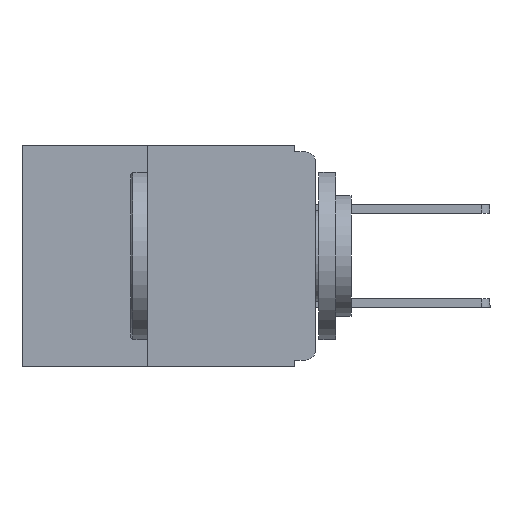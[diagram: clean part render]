
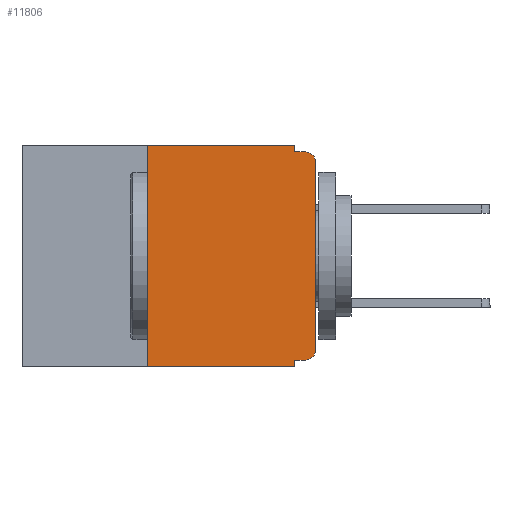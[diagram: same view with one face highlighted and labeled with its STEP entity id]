
A CAD part, left-side view. The second image highlights one B-rep face of the part: STEP entity #11806.
In plain terms, the highlighted planar face has unit normal (-1, 0, 0).
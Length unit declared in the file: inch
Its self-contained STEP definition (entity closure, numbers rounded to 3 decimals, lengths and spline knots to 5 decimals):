
#824 = EDGE_CURVE ( 'NONE', #16951, #5753, #6461, .T. ) ;
#980 = DIRECTION ( 'NONE',  ( 0., -1., 0. ) ) ;
#1070 = CARTESIAN_POINT ( 'NONE',  ( 0., 0., -0.305 ) ) ;
#1352 = EDGE_CURVE ( 'NONE', #15183, #16943, #2211, .T. ) ;
#1649 = VERTEX_POINT ( 'NONE', #15265 ) ;
#1796 = EDGE_CURVE ( 'NONE', #6173, #6223, #10322, .T. ) ;
#1927 = ORIENTED_EDGE ( 'NONE', *, *, #824, .F. ) ;
#2012 = VERTEX_POINT ( 'NONE', #11106 ) ;
#2022 = DIRECTION ( 'NONE',  ( 0., 0., -1. ) ) ;
#2211 = CIRCLE ( 'NONE', #7784, 0.015 ) ;
#2350 = VECTOR ( 'NONE', #8326, 39.37008 ) ;
#2513 = LINE ( 'NONE', #5973, #13495 ) ;
#2832 = VECTOR ( 'NONE', #980, 39.37008 ) ;
#3744 = EDGE_CURVE ( 'NONE', #2012, #5484, #15896, .T. ) ;
#3760 = ORIENTED_EDGE ( 'NONE', *, *, #16288, .F. ) ;
#3963 = ORIENTED_EDGE ( 'NONE', *, *, #9314, .F. ) ;
#4223 = CARTESIAN_POINT ( 'NONE',  ( 0., 0.437, -0.33 ) ) ;
#4314 = AXIS2_PLACEMENT_3D ( 'NONE', #6509, #6327, #6325 ) ;
#4913 = CARTESIAN_POINT ( 'NONE',  ( 0., 0.031, -0.32 ) ) ;
#5142 = ORIENTED_EDGE ( 'NONE', *, *, #7722, .F. ) ;
#5484 = VERTEX_POINT ( 'NONE', #10378 ) ;
#5493 = CARTESIAN_POINT ( 'NONE',  ( 0., 0., -0.32 ) ) ;
#5753 = VERTEX_POINT ( 'NONE', #10922 ) ;
#5779 = DIRECTION ( 'NONE',  ( 0., 0., 1. ) ) ;
#5806 = EDGE_CURVE ( 'NONE', #16943, #6173, #2513, .T. ) ;
#5818 = CARTESIAN_POINT ( 'NONE',  ( 0., 0.031, -0.33 ) ) ;
#5973 = CARTESIAN_POINT ( 'NONE',  ( 0., 0., 0. ) ) ;
#6000 = VECTOR ( 'NONE', #6075, 39.37008 ) ;
#6075 = DIRECTION ( 'NONE',  ( 0., 0., -1. ) ) ;
#6167 = VECTOR ( 'NONE', #16629, 39.37008 ) ;
#6173 = VERTEX_POINT ( 'NONE', #9390 ) ;
#6223 = VERTEX_POINT ( 'NONE', #9029 ) ;
#6226 = ORIENTED_EDGE ( 'NONE', *, *, #9392, .T. ) ;
#6325 = DIRECTION ( 'NONE',  ( 0., 0., -1. ) ) ;
#6327 = DIRECTION ( 'NONE',  ( -1., 0., 0. ) ) ;
#6461 = LINE ( 'NONE', #13357, #13639 ) ;
#6509 = CARTESIAN_POINT ( 'NONE',  ( 0., 0.015, -0.025 ) ) ;
#7722 = EDGE_CURVE ( 'NONE', #15510, #1649, #13208, .T. ) ;
#7759 = DIRECTION ( 'NONE',  ( -1., 0., 0. ) ) ;
#7763 = DIRECTION ( 'NONE',  ( 0., -1., 0. ) ) ;
#7784 = AXIS2_PLACEMENT_3D ( 'NONE', #17435, #7759, #12867 ) ;
#8326 = DIRECTION ( 'NONE',  ( 0., -1., 0. ) ) ;
#8402 = LINE ( 'NONE', #16883, #11637 ) ;
#8527 = ORIENTED_EDGE ( 'NONE', *, *, #13169, .F. ) ;
#8975 = AXIS2_PLACEMENT_3D ( 'NONE', #16760, #10423, #2022 ) ;
#9009 = PLANE ( 'NONE',  #8975 ) ;
#9029 = CARTESIAN_POINT ( 'NONE',  ( 0., 0.015, -0.01 ) ) ;
#9314 = EDGE_CURVE ( 'NONE', #15183, #15510, #14131, .T. ) ;
#9369 = LINE ( 'NONE', #4223, #2350 ) ;
#9372 = EDGE_LOOP ( 'NONE', ( #16491, #12739, #3760, #12754, #8527, #1927, #6226, #5142, #3963, #13866 ) ) ;
#9390 = CARTESIAN_POINT ( 'NONE',  ( 0., 0., -0.025 ) ) ;
#9392 = EDGE_CURVE ( 'NONE', #16951, #1649, #9369, .T. ) ;
#10322 = CIRCLE ( 'NONE', #4314, 0.015 ) ;
#10378 = CARTESIAN_POINT ( 'NONE',  ( 0., 0.031, -0.01 ) ) ;
#10423 = DIRECTION ( 'NONE',  ( 1., 0., 0. ) ) ;
#10922 = CARTESIAN_POINT ( 'NONE',  ( 0., 0.25, 0. ) ) ;
#11106 = CARTESIAN_POINT ( 'NONE',  ( 0., 0.031, 0. ) ) ;
#11637 = VECTOR ( 'NONE', #7763, 39.37008 ) ;
#11806 = ADVANCED_FACE ( 'NONE', ( #13460 ), #9009, .F. ) ;
#12739 = ORIENTED_EDGE ( 'NONE', *, *, #1796, .T. ) ;
#12754 = ORIENTED_EDGE ( 'NONE', *, *, #3744, .F. ) ;
#12867 = DIRECTION ( 'NONE',  ( 0., 0., -1. ) ) ;
#13169 = EDGE_CURVE ( 'NONE', #5753, #2012, #8402, .T. ) ;
#13208 = LINE ( 'NONE', #5818, #6000 ) ;
#13357 = CARTESIAN_POINT ( 'NONE',  ( 0., 0.25, -0.33 ) ) ;
#13460 = FACE_OUTER_BOUND ( 'NONE', #9372, .T. ) ;
#13495 = VECTOR ( 'NONE', #5779, 39.37008 ) ;
#13520 = CARTESIAN_POINT ( 'NONE',  ( 0., 0.25, -0.33 ) ) ;
#13635 = CARTESIAN_POINT ( 'NONE',  ( 0., 0.015, -0.32 ) ) ;
#13639 = VECTOR ( 'NONE', #15035, 39.37008 ) ;
#13866 = ORIENTED_EDGE ( 'NONE', *, *, #1352, .T. ) ;
#14131 = LINE ( 'NONE', #5493, #14523 ) ;
#14523 = VECTOR ( 'NONE', #16081, 39.37008 ) ;
#14626 = CARTESIAN_POINT ( 'NONE',  ( 0., 0., -0.01 ) ) ;
#15035 = DIRECTION ( 'NONE',  ( 0., 0., 1. ) ) ;
#15183 = VERTEX_POINT ( 'NONE', #13635 ) ;
#15265 = CARTESIAN_POINT ( 'NONE',  ( 0., 0.031, -0.33 ) ) ;
#15510 = VERTEX_POINT ( 'NONE', #4913 ) ;
#15896 = LINE ( 'NONE', #16328, #6167 ) ;
#16081 = DIRECTION ( 'NONE',  ( 0., 1., 0. ) ) ;
#16288 = EDGE_CURVE ( 'NONE', #5484, #6223, #17042, .T. ) ;
#16328 = CARTESIAN_POINT ( 'NONE',  ( 0., 0.031, 0. ) ) ;
#16491 = ORIENTED_EDGE ( 'NONE', *, *, #5806, .T. ) ;
#16629 = DIRECTION ( 'NONE',  ( 0., 0., -1. ) ) ;
#16760 = CARTESIAN_POINT ( 'NONE',  ( 0., 0.437, 0. ) ) ;
#16883 = CARTESIAN_POINT ( 'NONE',  ( 0., 0.437, 0. ) ) ;
#16943 = VERTEX_POINT ( 'NONE', #1070 ) ;
#16951 = VERTEX_POINT ( 'NONE', #13520 ) ;
#17042 = LINE ( 'NONE', #14626, #2832 ) ;
#17435 = CARTESIAN_POINT ( 'NONE',  ( 0., 0.015, -0.305 ) ) ;
